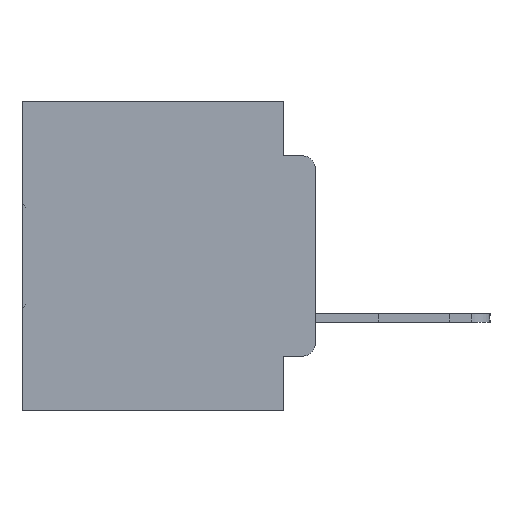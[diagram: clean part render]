
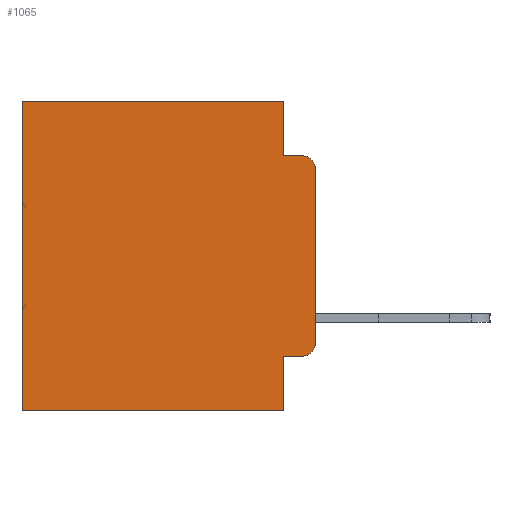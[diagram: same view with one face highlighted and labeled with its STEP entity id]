
A CAD part, left-side view. The second image highlights one B-rep face of the part: STEP entity #1065.
In plain terms, the highlighted planar face has unit normal (-1, 0, 0).
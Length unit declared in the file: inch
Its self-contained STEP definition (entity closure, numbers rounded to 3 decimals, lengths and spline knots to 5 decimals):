
#764 = DIRECTION ( 'NONE',  ( 0., -1., 0. ) ) ;
#1065 = ADVANCED_FACE ( 'NONE', ( #29598 ), #32862, .F. ) ;
#1544 = VERTEX_POINT ( 'NONE', #27838 ) ;
#1827 = CARTESIAN_POINT ( 'NONE',  ( 0.298, 0.02, -0.1085 ) ) ;
#2107 = CARTESIAN_POINT ( 'NONE',  ( 0.298, 0.051, 0. ) ) ;
#2632 = CIRCLE ( 'NONE', #13992, 0.02 ) ;
#2916 = VERTEX_POINT ( 'NONE', #7134 ) ;
#2992 = EDGE_CURVE ( 'NONE', #17109, #12213, #13576, .T. ) ;
#3071 = VECTOR ( 'NONE', #6017, 39.37008 ) ;
#3339 = CARTESIAN_POINT ( 'NONE',  ( 0.298, 0.051, -0.0885 ) ) ;
#3844 = ORIENTED_EDGE ( 'NONE', *, *, #2992, .F. ) ;
#3932 = VERTEX_POINT ( 'NONE', #21344 ) ;
#4064 = VERTEX_POINT ( 'NONE', #26968 ) ;
#4124 = CARTESIAN_POINT ( 'NONE',  ( 0.298, 0.473, 0. ) ) ;
#4573 = DIRECTION ( 'NONE',  ( 0., 0., -1. ) ) ;
#4857 = DIRECTION ( 'NONE',  ( 0., 0., -1. ) ) ;
#5064 = VECTOR ( 'NONE', #21936, 39.37008 ) ;
#6017 = DIRECTION ( 'NONE',  ( 0., -1., 0. ) ) ;
#6401 = LINE ( 'NONE', #24227, #32611 ) ;
#6414 = CARTESIAN_POINT ( 'NONE',  ( 0.298, 0.02, -0.3915 ) ) ;
#6729 = VECTOR ( 'NONE', #26457, 39.37008 ) ;
#7134 = CARTESIAN_POINT ( 'NONE',  ( 0.298, 0.02, -0.4115 ) ) ;
#7223 = VECTOR ( 'NONE', #32209, 39.37008 ) ;
#7451 = CARTESIAN_POINT ( 'NONE',  ( 0.298, 0.051, 0. ) ) ;
#8962 = ORIENTED_EDGE ( 'NONE', *, *, #19313, .T. ) ;
#9036 = DIRECTION ( 'NONE',  ( 0., 0., -1. ) ) ;
#9390 = LINE ( 'NONE', #2107, #22238 ) ;
#9412 = ORIENTED_EDGE ( 'NONE', *, *, #9416, .F. ) ;
#9416 = EDGE_CURVE ( 'NONE', #4064, #9694, #6401, .T. ) ;
#9694 = VERTEX_POINT ( 'NONE', #15057 ) ;
#10891 = VERTEX_POINT ( 'NONE', #25540 ) ;
#11946 = LINE ( 'NONE', #26879, #5064 ) ;
#12108 = VECTOR ( 'NONE', #25337, 39.37008 ) ;
#12213 = VERTEX_POINT ( 'NONE', #12427 ) ;
#12427 = CARTESIAN_POINT ( 'NONE',  ( 0.298, 0., -0.3915 ) ) ;
#12505 = CARTESIAN_POINT ( 'NONE',  ( 0.298, 0.02, -0.0885 ) ) ;
#13062 = ORIENTED_EDGE ( 'NONE', *, *, #29438, .T. ) ;
#13282 = EDGE_CURVE ( 'NONE', #29923, #1544, #11946, .T. ) ;
#13576 = LINE ( 'NONE', #26500, #6729 ) ;
#13584 = ORIENTED_EDGE ( 'NONE', *, *, #22704, .T. ) ;
#13992 = AXIS2_PLACEMENT_3D ( 'NONE', #6414, #24352, #9036 ) ;
#14066 = LINE ( 'NONE', #4124, #7223 ) ;
#15057 = CARTESIAN_POINT ( 'NONE',  ( 0.298, 0.473, -0.5 ) ) ;
#16659 = EDGE_LOOP ( 'NONE', ( #3844, #13062, #32007, #28747, #32625, #13584, #9412, #32057, #8962, #17764 ) ) ;
#16698 = VECTOR ( 'NONE', #764, 39.37008 ) ;
#17109 = VERTEX_POINT ( 'NONE', #23115 ) ;
#17603 = EDGE_CURVE ( 'NONE', #2916, #12213, #2632, .T. ) ;
#17764 = ORIENTED_EDGE ( 'NONE', *, *, #17603, .T. ) ;
#17932 = CIRCLE ( 'NONE', #31631, 0.02 ) ;
#19313 = EDGE_CURVE ( 'NONE', #3932, #2916, #30125, .T. ) ;
#20055 = DIRECTION ( 'NONE',  ( -1., 0., 0. ) ) ;
#21025 = EDGE_CURVE ( 'NONE', #3932, #4064, #31552, .T. ) ;
#21344 = CARTESIAN_POINT ( 'NONE',  ( 0.298, 0.051, -0.4115 ) ) ;
#21809 = DIRECTION ( 'NONE',  ( 0., 1., 0. ) ) ;
#21936 = DIRECTION ( 'NONE',  ( 0., 1., 0. ) ) ;
#22238 = VECTOR ( 'NONE', #4857, 39.37008 ) ;
#22704 = EDGE_CURVE ( 'NONE', #1544, #9694, #14066, .T. ) ;
#23115 = CARTESIAN_POINT ( 'NONE',  ( 0.298, 0., -0.1085 ) ) ;
#23675 = LINE ( 'NONE', #3339, #3071 ) ;
#24227 = CARTESIAN_POINT ( 'NONE',  ( 0.298, 0., -0.5 ) ) ;
#24352 = DIRECTION ( 'NONE',  ( -1., 0., 0. ) ) ;
#24412 = EDGE_CURVE ( 'NONE', #29923, #10891, #9390, .T. ) ;
#25337 = DIRECTION ( 'NONE',  ( 0., 0., -1. ) ) ;
#25540 = CARTESIAN_POINT ( 'NONE',  ( 0.298, 0.051, -0.0885 ) ) ;
#26081 = EDGE_CURVE ( 'NONE', #10891, #26927, #23675, .T. ) ;
#26457 = DIRECTION ( 'NONE',  ( 0., 0., -1. ) ) ;
#26500 = CARTESIAN_POINT ( 'NONE',  ( 0.298, 0., 0. ) ) ;
#26879 = CARTESIAN_POINT ( 'NONE',  ( 0.298, 0., 0. ) ) ;
#26927 = VERTEX_POINT ( 'NONE', #12505 ) ;
#26968 = CARTESIAN_POINT ( 'NONE',  ( 0.298, 0.051, -0.5 ) ) ;
#27838 = CARTESIAN_POINT ( 'NONE',  ( 0.298, 0.473, 0. ) ) ;
#28747 = ORIENTED_EDGE ( 'NONE', *, *, #24412, .F. ) ;
#29281 = CARTESIAN_POINT ( 'NONE',  ( 0.298, 0.051, 0. ) ) ;
#29438 = EDGE_CURVE ( 'NONE', #17109, #26927, #17932, .T. ) ;
#29598 = FACE_OUTER_BOUND ( 'NONE', #16659, .T. ) ;
#29923 = VERTEX_POINT ( 'NONE', #29281 ) ;
#30125 = LINE ( 'NONE', #31567, #16698 ) ;
#30251 = AXIS2_PLACEMENT_3D ( 'NONE', #32659, #32448, #32217 ) ;
#31552 = LINE ( 'NONE', #7451, #12108 ) ;
#31567 = CARTESIAN_POINT ( 'NONE',  ( 0.298, 0.051, -0.4115 ) ) ;
#31631 = AXIS2_PLACEMENT_3D ( 'NONE', #1827, #20055, #4573 ) ;
#32007 = ORIENTED_EDGE ( 'NONE', *, *, #26081, .F. ) ;
#32057 = ORIENTED_EDGE ( 'NONE', *, *, #21025, .F. ) ;
#32209 = DIRECTION ( 'NONE',  ( 0., 0., -1. ) ) ;
#32217 = DIRECTION ( 'NONE',  ( 0., 0., -1. ) ) ;
#32448 = DIRECTION ( 'NONE',  ( 1., 0., 0. ) ) ;
#32611 = VECTOR ( 'NONE', #21809, 39.37008 ) ;
#32625 = ORIENTED_EDGE ( 'NONE', *, *, #13282, .T. ) ;
#32659 = CARTESIAN_POINT ( 'NONE',  ( 0.298, 0., 0. ) ) ;
#32862 = PLANE ( 'NONE',  #30251 ) ;
